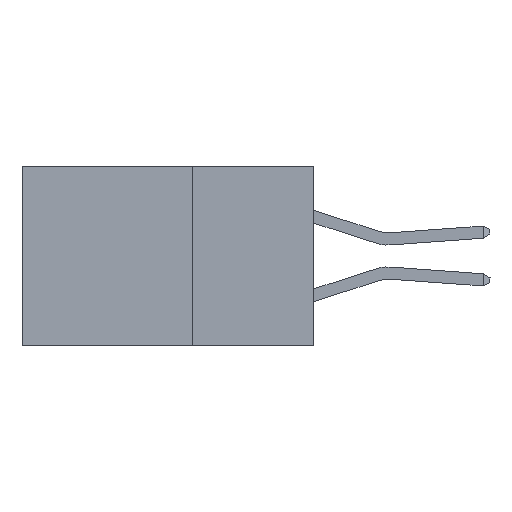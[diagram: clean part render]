
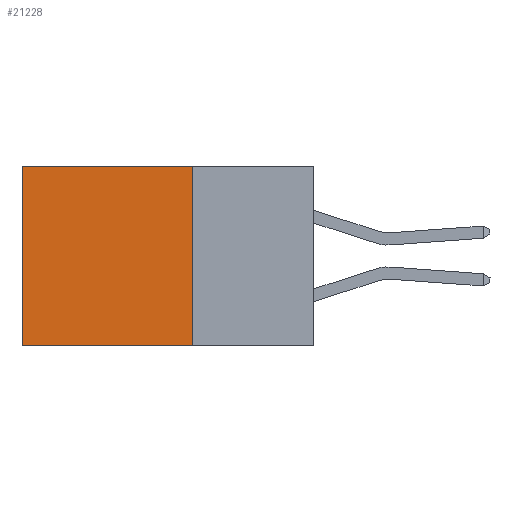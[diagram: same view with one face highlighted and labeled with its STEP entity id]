
A CAD part, left-side view. The second image highlights one B-rep face of the part: STEP entity #21228.
In plain terms, the highlighted planar face has unit normal (-1, 0, 0).
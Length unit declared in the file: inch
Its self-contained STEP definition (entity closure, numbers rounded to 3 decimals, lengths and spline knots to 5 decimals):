
#515 = LINE ( 'NONE', #21783, #2932 ) ;
#1185 = CARTESIAN_POINT ( 'NONE',  ( 0.2875, 0.6, 0. ) ) ;
#1238 = EDGE_CURVE ( 'NONE', #11556, #21220, #515, .T. ) ;
#1505 = CARTESIAN_POINT ( 'NONE',  ( 0.2875, 0.6, -0.37 ) ) ;
#2049 = VERTEX_POINT ( 'NONE', #1505 ) ;
#2729 = AXIS2_PLACEMENT_3D ( 'NONE', #31191, #7514, #17072 ) ;
#2771 = DIRECTION ( 'NONE',  ( 0., 1., 0. ) ) ;
#2932 = VECTOR ( 'NONE', #2771, 39.37008 ) ;
#4507 = ORIENTED_EDGE ( 'NONE', *, *, #1238, .T. ) ;
#6245 = DIRECTION ( 'NONE',  ( 0., 0., -1. ) ) ;
#7514 = DIRECTION ( 'NONE',  ( 1., 0., 0. ) ) ;
#8169 = EDGE_CURVE ( 'NONE', #11556, #13957, #29880, .T. ) ;
#8265 = CARTESIAN_POINT ( 'NONE',  ( 0.2875, 0.25, 0. ) ) ;
#9522 = EDGE_CURVE ( 'NONE', #21220, #2049, #21808, .T. ) ;
#11556 = VERTEX_POINT ( 'NONE', #16354 ) ;
#13957 = VERTEX_POINT ( 'NONE', #27172 ) ;
#14188 = CARTESIAN_POINT ( 'NONE',  ( 0.2875, 0.6, 0. ) ) ;
#15285 = FACE_OUTER_BOUND ( 'NONE', #26378, .T. ) ;
#16354 = CARTESIAN_POINT ( 'NONE',  ( 0.2875, 0.25, 0. ) ) ;
#17072 = DIRECTION ( 'NONE',  ( 0., 0., -1. ) ) ;
#18821 = DIRECTION ( 'NONE',  ( 0., 0., -1. ) ) ;
#20663 = PLANE ( 'NONE',  #2729 ) ;
#21202 = VECTOR ( 'NONE', #18821, 39.37008 ) ;
#21220 = VERTEX_POINT ( 'NONE', #1185 ) ;
#21228 = ADVANCED_FACE ( 'NONE', ( #15285 ), #20663, .F. ) ;
#21783 = CARTESIAN_POINT ( 'NONE',  ( 0.2875, 0.25, 0. ) ) ;
#21808 = LINE ( 'NONE', #14188, #32283 ) ;
#25248 = ORIENTED_EDGE ( 'NONE', *, *, #25376, .F. ) ;
#25376 = EDGE_CURVE ( 'NONE', #13957, #2049, #29114, .T. ) ;
#26378 = EDGE_LOOP ( 'NONE', ( #27122, #25248, #29928, #4507 ) ) ;
#27122 = ORIENTED_EDGE ( 'NONE', *, *, #9522, .T. ) ;
#27172 = CARTESIAN_POINT ( 'NONE',  ( 0.2875, 0.25, -0.37 ) ) ;
#28434 = CARTESIAN_POINT ( 'NONE',  ( 0.2875, 0.25, -0.37 ) ) ;
#29114 = LINE ( 'NONE', #28434, #32657 ) ;
#29880 = LINE ( 'NONE', #8265, #21202 ) ;
#29928 = ORIENTED_EDGE ( 'NONE', *, *, #8169, .F. ) ;
#31191 = CARTESIAN_POINT ( 'NONE',  ( 0.2875, 0.25, 0. ) ) ;
#31363 = DIRECTION ( 'NONE',  ( 0., 1., 0. ) ) ;
#32283 = VECTOR ( 'NONE', #6245, 39.37008 ) ;
#32657 = VECTOR ( 'NONE', #31363, 39.37008 ) ;
